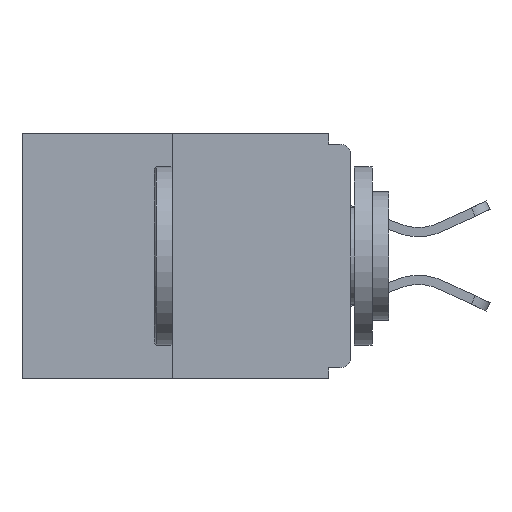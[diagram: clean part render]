
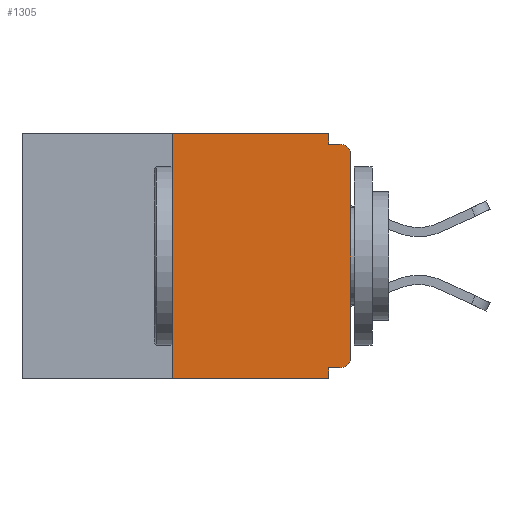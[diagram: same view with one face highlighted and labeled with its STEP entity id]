
A CAD part, left-side view. The second image highlights one B-rep face of the part: STEP entity #1305.
In plain terms, the highlighted planar face has unit normal (-1, 0, 0).
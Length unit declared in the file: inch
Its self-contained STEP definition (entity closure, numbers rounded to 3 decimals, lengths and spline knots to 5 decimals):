
#108 = DIRECTION ( 'NONE',  ( -1., 0., 0. ) ) ;
#335 = VECTOR ( 'NONE', #4049, 39.37008 ) ;
#1305 = ADVANCED_FACE ( 'NONE', ( #17199 ), #23863, .F. ) ;
#2618 = CARTESIAN_POINT ( 'NONE',  ( 0., 0.031, -0.328 ) ) ;
#2726 = VERTEX_POINT ( 'NONE', #2618 ) ;
#2910 = ORIENTED_EDGE ( 'NONE', *, *, #19755, .T. ) ;
#2946 = CARTESIAN_POINT ( 'NONE',  ( 0., 0.031, -0.015 ) ) ;
#3057 = CARTESIAN_POINT ( 'NONE',  ( 0., 0., -0.015 ) ) ;
#3404 = VERTEX_POINT ( 'NONE', #2946 ) ;
#3427 = ORIENTED_EDGE ( 'NONE', *, *, #26045, .F. ) ;
#3909 = DIRECTION ( 'NONE',  ( 0., 0., 1. ) ) ;
#4049 = DIRECTION ( 'NONE',  ( 0., -1., 0. ) ) ;
#4196 = AXIS2_PLACEMENT_3D ( 'NONE', #5827, #14300, #18649 ) ;
#4490 = EDGE_CURVE ( 'NONE', #11435, #3404, #26707, .T. ) ;
#4499 = CIRCLE ( 'NONE', #4196, 0.015 ) ;
#4540 = VECTOR ( 'NONE', #5901, 39.37008 ) ;
#4650 = AXIS2_PLACEMENT_3D ( 'NONE', #8586, #108, #19427 ) ;
#4734 = EDGE_CURVE ( 'NONE', #2726, #23643, #5029, .T. ) ;
#5014 = CARTESIAN_POINT ( 'NONE',  ( 0., 0.031, -0.343 ) ) ;
#5029 = LINE ( 'NONE', #5014, #15718 ) ;
#5188 = VERTEX_POINT ( 'NONE', #27010 ) ;
#5396 = EDGE_LOOP ( 'NONE', ( #3427, #15849, #24272, #26390, #20714, #14027, #11788, #2910, #18373, #9042 ) ) ;
#5800 = DIRECTION ( 'NONE',  ( 0., 0., -1. ) ) ;
#5827 = CARTESIAN_POINT ( 'NONE',  ( 0., 0.015, -0.313 ) ) ;
#5854 = VERTEX_POINT ( 'NONE', #25175 ) ;
#5901 = DIRECTION ( 'NONE',  ( 0., -1., 0. ) ) ;
#6175 = CARTESIAN_POINT ( 'NONE',  ( 0., 0., -0.313 ) ) ;
#6519 = LINE ( 'NONE', #7028, #18476 ) ;
#6661 = DIRECTION ( 'NONE',  ( 0., 0., 1. ) ) ;
#7028 = CARTESIAN_POINT ( 'NONE',  ( 0., 0.25, 0. ) ) ;
#7709 = EDGE_CURVE ( 'NONE', #18809, #23643, #23318, .T. ) ;
#8176 = LINE ( 'NONE', #23364, #22469 ) ;
#8586 = CARTESIAN_POINT ( 'NONE',  ( 0., 0.015, -0.03 ) ) ;
#8864 = DIRECTION ( 'NONE',  ( 0., 1., 0. ) ) ;
#9042 = ORIENTED_EDGE ( 'NONE', *, *, #4490, .F. ) ;
#9329 = DIRECTION ( 'NONE',  ( 0., 0., -1. ) ) ;
#10896 = CARTESIAN_POINT ( 'NONE',  ( 0., 0.25, -0.343 ) ) ;
#11061 = EDGE_CURVE ( 'NONE', #19074, #5188, #20092, .T. ) ;
#11435 = VERTEX_POINT ( 'NONE', #22923 ) ;
#11788 = ORIENTED_EDGE ( 'NONE', *, *, #11061, .T. ) ;
#12481 = CIRCLE ( 'NONE', #4650, 0.015 ) ;
#12925 = CARTESIAN_POINT ( 'NONE',  ( 0., 0.46, 0. ) ) ;
#13196 = DIRECTION ( 'NONE',  ( 1., 0., 0. ) ) ;
#13378 = EDGE_CURVE ( 'NONE', #5854, #19074, #4499, .T. ) ;
#13780 = EDGE_CURVE ( 'NONE', #18809, #18808, #6519, .T. ) ;
#13832 = VECTOR ( 'NONE', #3909, 39.37008 ) ;
#14027 = ORIENTED_EDGE ( 'NONE', *, *, #13378, .T. ) ;
#14161 = EDGE_CURVE ( 'NONE', #5854, #2726, #8176, .T. ) ;
#14300 = DIRECTION ( 'NONE',  ( -1., 0., 0. ) ) ;
#15501 = DIRECTION ( 'NONE',  ( 0., -1., 0. ) ) ;
#15718 = VECTOR ( 'NONE', #9329, 39.37008 ) ;
#15849 = ORIENTED_EDGE ( 'NONE', *, *, #13780, .F. ) ;
#16005 = CARTESIAN_POINT ( 'NONE',  ( 0., 0.015, -0.015 ) ) ;
#16018 = AXIS2_PLACEMENT_3D ( 'NONE', #12925, #13196, #21426 ) ;
#16309 = LINE ( 'NONE', #3057, #19272 ) ;
#16579 = CARTESIAN_POINT ( 'NONE',  ( 0., 0.031, 0. ) ) ;
#16694 = CARTESIAN_POINT ( 'NONE',  ( 0., 0., 0. ) ) ;
#16832 = CARTESIAN_POINT ( 'NONE',  ( 0., 0.46, -0.343 ) ) ;
#17199 = FACE_OUTER_BOUND ( 'NONE', #5396, .T. ) ;
#18373 = ORIENTED_EDGE ( 'NONE', *, *, #23078, .F. ) ;
#18476 = VECTOR ( 'NONE', #6661, 39.37008 ) ;
#18628 = CARTESIAN_POINT ( 'NONE',  ( 0., 0.46, 0. ) ) ;
#18649 = DIRECTION ( 'NONE',  ( 0., 0., -1. ) ) ;
#18808 = VERTEX_POINT ( 'NONE', #21548 ) ;
#18809 = VERTEX_POINT ( 'NONE', #10896 ) ;
#19074 = VERTEX_POINT ( 'NONE', #6175 ) ;
#19272 = VECTOR ( 'NONE', #15501, 39.37008 ) ;
#19427 = DIRECTION ( 'NONE',  ( 0., 0., -1. ) ) ;
#19755 = EDGE_CURVE ( 'NONE', #5188, #24603, #12481, .T. ) ;
#20092 = LINE ( 'NONE', #16694, #13832 ) ;
#20714 = ORIENTED_EDGE ( 'NONE', *, *, #14161, .F. ) ;
#21426 = DIRECTION ( 'NONE',  ( 0., 0., -1. ) ) ;
#21548 = CARTESIAN_POINT ( 'NONE',  ( 0., 0.25, 0. ) ) ;
#22469 = VECTOR ( 'NONE', #8864, 39.37008 ) ;
#22703 = VECTOR ( 'NONE', #5800, 39.37008 ) ;
#22923 = CARTESIAN_POINT ( 'NONE',  ( 0., 0.031, 0. ) ) ;
#23078 = EDGE_CURVE ( 'NONE', #3404, #24603, #16309, .T. ) ;
#23318 = LINE ( 'NONE', #16832, #335 ) ;
#23364 = CARTESIAN_POINT ( 'NONE',  ( 0., 0., -0.328 ) ) ;
#23643 = VERTEX_POINT ( 'NONE', #23943 ) ;
#23863 = PLANE ( 'NONE',  #16018 ) ;
#23943 = CARTESIAN_POINT ( 'NONE',  ( 0., 0.031, -0.343 ) ) ;
#24272 = ORIENTED_EDGE ( 'NONE', *, *, #7709, .T. ) ;
#24603 = VERTEX_POINT ( 'NONE', #16005 ) ;
#25175 = CARTESIAN_POINT ( 'NONE',  ( 0., 0.015, -0.328 ) ) ;
#25530 = LINE ( 'NONE', #18628, #4540 ) ;
#26045 = EDGE_CURVE ( 'NONE', #18808, #11435, #25530, .T. ) ;
#26390 = ORIENTED_EDGE ( 'NONE', *, *, #4734, .F. ) ;
#26707 = LINE ( 'NONE', #16579, #22703 ) ;
#27010 = CARTESIAN_POINT ( 'NONE',  ( 0., 0., -0.03 ) ) ;
